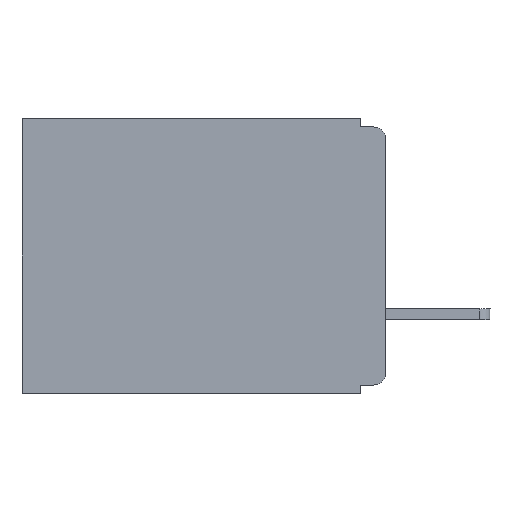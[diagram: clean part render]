
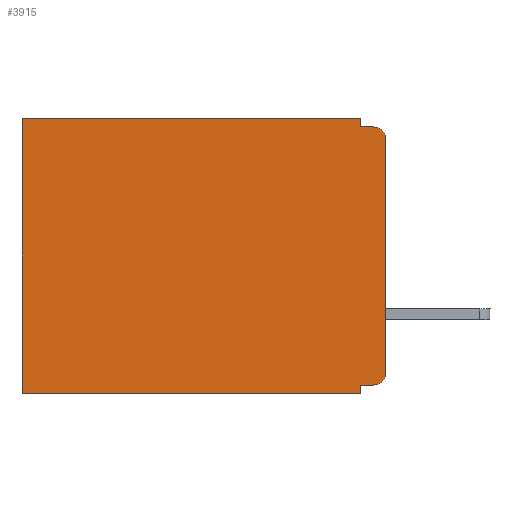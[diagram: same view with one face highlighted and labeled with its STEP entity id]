
A CAD part, left-side view. The second image highlights one B-rep face of the part: STEP entity #3915.
In plain terms, the highlighted planar face has unit normal (-1, 0, 0).
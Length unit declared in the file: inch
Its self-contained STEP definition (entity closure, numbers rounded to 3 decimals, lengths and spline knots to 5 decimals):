
#207 = DIRECTION ( 'NONE',  ( 1., 0., 0. ) ) ;
#231 = VERTEX_POINT ( 'NONE', #6378 ) ;
#310 = DIRECTION ( 'NONE',  ( 0., 0., -1. ) ) ;
#331 = CARTESIAN_POINT ( 'NONE',  ( 0.3, 0., -0.32 ) ) ;
#675 = CARTESIAN_POINT ( 'NONE',  ( 0.3, 0.031, 0. ) ) ;
#707 = CARTESIAN_POINT ( 'NONE',  ( 0.3, 0., -0.305 ) ) ;
#853 = AXIS2_PLACEMENT_3D ( 'NONE', #8861, #3271, #8962 ) ;
#1028 = CARTESIAN_POINT ( 'NONE',  ( 0.3, 0.437, -0.33 ) ) ;
#1123 = DIRECTION ( 'NONE',  ( 0., -1., 0. ) ) ;
#1172 = EDGE_CURVE ( 'NONE', #10511, #3897, #9861, .T. ) ;
#1565 = EDGE_CURVE ( 'NONE', #3485, #7193, #5015, .T. ) ;
#2008 = CARTESIAN_POINT ( 'NONE',  ( 0.3, 0.031, -0.01 ) ) ;
#2105 = EDGE_CURVE ( 'NONE', #9596, #10422, #5334, .T. ) ;
#2120 = CARTESIAN_POINT ( 'NONE',  ( 0.3, 0., -0.33 ) ) ;
#2642 = AXIS2_PLACEMENT_3D ( 'NONE', #5206, #207, #310 ) ;
#2667 = DIRECTION ( 'NONE',  ( 0., 0., -1. ) ) ;
#2681 = ORIENTED_EDGE ( 'NONE', *, *, #2853, .F. ) ;
#2686 = EDGE_CURVE ( 'NONE', #9491, #7193, #8838, .T. ) ;
#2721 = PLANE ( 'NONE',  #2642 ) ;
#2853 = EDGE_CURVE ( 'NONE', #6623, #10511, #7921, .T. ) ;
#3127 = DIRECTION ( 'NONE',  ( 0., 0., -1. ) ) ;
#3196 = CIRCLE ( 'NONE', #7754, 0.015 ) ;
#3271 = DIRECTION ( 'NONE',  ( -1., 0., 0. ) ) ;
#3411 = VECTOR ( 'NONE', #8747, 39.37008 ) ;
#3484 = VECTOR ( 'NONE', #1123, 39.37008 ) ;
#3485 = VERTEX_POINT ( 'NONE', #6099 ) ;
#3679 = EDGE_CURVE ( 'NONE', #231, #9491, #7902, .T. ) ;
#3748 = CARTESIAN_POINT ( 'NONE',  ( 0.3, 0.015, -0.01 ) ) ;
#3770 = EDGE_CURVE ( 'NONE', #3897, #10422, #4609, .T. ) ;
#3810 = DIRECTION ( 'NONE',  ( 0., 0., -1. ) ) ;
#3848 = EDGE_CURVE ( 'NONE', #6623, #8129, #3196, .T. ) ;
#3897 = VERTEX_POINT ( 'NONE', #6859 ) ;
#3915 = ADVANCED_FACE ( 'NONE', ( #7636 ), #2721, .F. ) ;
#3978 = ORIENTED_EDGE ( 'NONE', *, *, #3848, .T. ) ;
#4050 = LINE ( 'NONE', #5587, #3411 ) ;
#4609 = LINE ( 'NONE', #5755, #8045 ) ;
#5015 = CIRCLE ( 'NONE', #853, 0.015 ) ;
#5108 = CARTESIAN_POINT ( 'NONE',  ( 0.3, 0., -0.01 ) ) ;
#5206 = CARTESIAN_POINT ( 'NONE',  ( 0.3, 0., -0.33 ) ) ;
#5287 = EDGE_CURVE ( 'NONE', #231, #9596, #4050, .T. ) ;
#5315 = VECTOR ( 'NONE', #3810, 39.37008 ) ;
#5334 = LINE ( 'NONE', #1028, #10142 ) ;
#5427 = VECTOR ( 'NONE', #2667, 39.37008 ) ;
#5474 = ORIENTED_EDGE ( 'NONE', *, *, #1565, .T. ) ;
#5547 = ORIENTED_EDGE ( 'NONE', *, *, #6974, .F. ) ;
#5587 = CARTESIAN_POINT ( 'NONE',  ( 0.3, 0., 0. ) ) ;
#5755 = CARTESIAN_POINT ( 'NONE',  ( 0.3, 0., -0.33 ) ) ;
#6052 = CARTESIAN_POINT ( 'NONE',  ( 0.3, 0.015, -0.305 ) ) ;
#6099 = CARTESIAN_POINT ( 'NONE',  ( 0.3, 0., -0.025 ) ) ;
#6378 = CARTESIAN_POINT ( 'NONE',  ( 0.3, 0.031, 0. ) ) ;
#6623 = VERTEX_POINT ( 'NONE', #7294 ) ;
#6814 = DIRECTION ( 'NONE',  ( 0., 1., 0. ) ) ;
#6859 = CARTESIAN_POINT ( 'NONE',  ( 0.3, 0.031, -0.33 ) ) ;
#6882 = CARTESIAN_POINT ( 'NONE',  ( 0.3, 0.031, -0.32 ) ) ;
#6974 = EDGE_CURVE ( 'NONE', #3485, #8129, #10131, .T. ) ;
#7042 = CARTESIAN_POINT ( 'NONE',  ( 0.3, 0.437, 0. ) ) ;
#7193 = VERTEX_POINT ( 'NONE', #3748 ) ;
#7294 = CARTESIAN_POINT ( 'NONE',  ( 0.3, 0.015, -0.32 ) ) ;
#7386 = ORIENTED_EDGE ( 'NONE', *, *, #5287, .T. ) ;
#7457 = DIRECTION ( 'NONE',  ( 0., 1., 0. ) ) ;
#7570 = DIRECTION ( 'NONE',  ( 0., 0., -1. ) ) ;
#7620 = DIRECTION ( 'NONE',  ( 0., 0., -1. ) ) ;
#7636 = FACE_OUTER_BOUND ( 'NONE', #8655, .T. ) ;
#7754 = AXIS2_PLACEMENT_3D ( 'NONE', #6052, #9239, #7620 ) ;
#7902 = LINE ( 'NONE', #675, #9819 ) ;
#7915 = ORIENTED_EDGE ( 'NONE', *, *, #1172, .F. ) ;
#7921 = LINE ( 'NONE', #331, #8055 ) ;
#8045 = VECTOR ( 'NONE', #7457, 39.37008 ) ;
#8055 = VECTOR ( 'NONE', #6814, 39.37008 ) ;
#8129 = VERTEX_POINT ( 'NONE', #707 ) ;
#8200 = CARTESIAN_POINT ( 'NONE',  ( 0.3, 0.437, -0.33 ) ) ;
#8438 = CARTESIAN_POINT ( 'NONE',  ( 0.3, 0.031, -0.33 ) ) ;
#8511 = ORIENTED_EDGE ( 'NONE', *, *, #3679, .F. ) ;
#8655 = EDGE_LOOP ( 'NONE', ( #5547, #5474, #8885, #8511, #7386, #9808, #9282, #7915, #2681, #3978 ) ) ;
#8747 = DIRECTION ( 'NONE',  ( 0., 1., 0. ) ) ;
#8838 = LINE ( 'NONE', #5108, #3484 ) ;
#8861 = CARTESIAN_POINT ( 'NONE',  ( 0.3, 0.015, -0.025 ) ) ;
#8885 = ORIENTED_EDGE ( 'NONE', *, *, #2686, .F. ) ;
#8962 = DIRECTION ( 'NONE',  ( 0., 0., -1. ) ) ;
#9239 = DIRECTION ( 'NONE',  ( -1., 0., 0. ) ) ;
#9282 = ORIENTED_EDGE ( 'NONE', *, *, #3770, .F. ) ;
#9491 = VERTEX_POINT ( 'NONE', #2008 ) ;
#9596 = VERTEX_POINT ( 'NONE', #7042 ) ;
#9808 = ORIENTED_EDGE ( 'NONE', *, *, #2105, .T. ) ;
#9819 = VECTOR ( 'NONE', #3127, 39.37008 ) ;
#9861 = LINE ( 'NONE', #8438, #5427 ) ;
#10131 = LINE ( 'NONE', #2120, #5315 ) ;
#10142 = VECTOR ( 'NONE', #7570, 39.37008 ) ;
#10422 = VERTEX_POINT ( 'NONE', #8200 ) ;
#10511 = VERTEX_POINT ( 'NONE', #6882 ) ;
